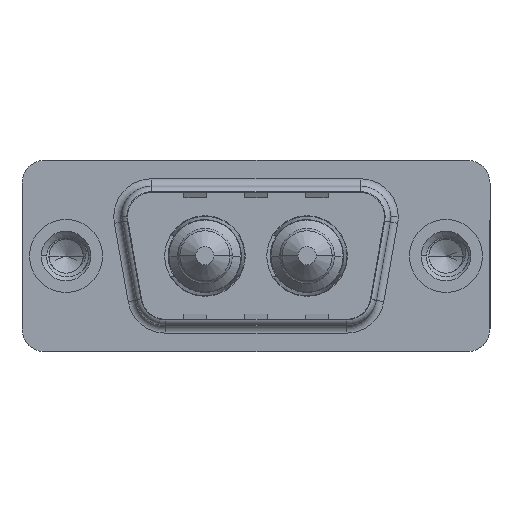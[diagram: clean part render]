
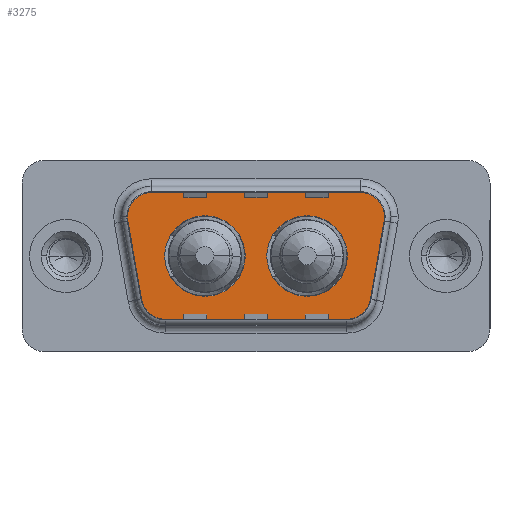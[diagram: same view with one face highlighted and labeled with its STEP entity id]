
A CAD part, top view. The second image highlights one B-rep face of the part: STEP entity #3275.
In plain terms, the highlighted planar face has unit normal (0, 0, 1).
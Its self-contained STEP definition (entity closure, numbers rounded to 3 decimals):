
#17 = EDGE_CURVE ( 'NONE', #4552, #8587, #10843, .T. ) ;
#69 = VECTOR ( 'NONE', #9359, 1000. ) ;
#136 = DIRECTION ( 'NONE',  ( 0., 0., 1. ) ) ;
#342 = CARTESIAN_POINT ( 'NONE',  ( 21.534, 2.553, 0. ) ) ;
#402 = VERTEX_POINT ( 'NONE', #11069 ) ;
#480 = DIRECTION ( 'NONE',  ( -1., 0., 0. ) ) ;
#673 = DIRECTION ( 'NONE',  ( 0.174, -0.985, 0. ) ) ;
#839 = EDGE_CURVE ( 'NONE', #10419, #3076, #1350, .T. ) ;
#845 = ORIENTED_EDGE ( 'NONE', *, *, #6918, .F. ) ;
#943 = CARTESIAN_POINT ( 'NONE',  ( 11.79, 0., 0. ) ) ;
#993 = CARTESIAN_POINT ( 'NONE',  ( 19.564, 2.9, 0. ) ) ;
#1350 = CIRCLE ( 'NONE', #9369, 2. ) ;
#1562 = FACE_BOUND ( 'NONE', #8953, .T. ) ;
#1615 = CARTESIAN_POINT ( 'NONE',  ( 18.541, -4.9, 0. ) ) ;
#1668 = VERTEX_POINT ( 'NONE', #3871 ) ;
#1776 = AXIS2_PLACEMENT_3D ( 'NONE', #9041, #3293, #10035 ) ;
#1849 = CARTESIAN_POINT ( 'NONE',  ( 19.564, 2.9, 0. ) ) ;
#1935 = DIRECTION ( 'NONE',  ( 0., 0., 1. ) ) ;
#1953 = DIRECTION ( 'NONE',  ( 0., 0., 1. ) ) ;
#1958 = DIRECTION ( 'NONE',  ( -1., 0., 0. ) ) ;
#2004 = VECTOR ( 'NONE', #673, 1000. ) ;
#2191 = CARTESIAN_POINT ( 'NONE',  ( 21.564, 2.9, 0. ) ) ;
#2252 = DIRECTION ( 'NONE',  ( 1., 0., 0. ) ) ;
#2276 = LINE ( 'NONE', #2548, #2004 ) ;
#2434 = PLANE ( 'NONE',  #11104 ) ;
#2440 = EDGE_CURVE ( 'NONE', #1668, #12020, #4058, .T. ) ;
#2451 = CARTESIAN_POINT ( 'NONE',  ( 5.436, 2.9, 0. ) ) ;
#2518 = CARTESIAN_POINT ( 'NONE',  ( 13.21, 0., 0. ) ) ;
#2548 = CARTESIAN_POINT ( 'NONE',  ( 3.466, 2.553, 0. ) ) ;
#2599 = EDGE_CURVE ( 'NONE', #3183, #10419, #2601, .T. ) ;
#2601 = LINE ( 'NONE', #342, #69 ) ;
#2719 = EDGE_LOOP ( 'NONE', ( #7186, #10573 ) ) ;
#2853 = EDGE_CURVE ( 'NONE', #3984, #3183, #10420, .T. ) ;
#2894 = VECTOR ( 'NONE', #6659, 1000. ) ;
#3076 = VERTEX_POINT ( 'NONE', #2191 ) ;
#3104 = ORIENTED_EDGE ( 'NONE', *, *, #2440, .T. ) ;
#3174 = LINE ( 'NONE', #8544, #2894 ) ;
#3183 = VERTEX_POINT ( 'NONE', #6648 ) ;
#3245 = DIRECTION ( 'NONE',  ( 0., 0., 1. ) ) ;
#3275 = ADVANCED_FACE ( 'NONE', ( #6599, #1562, #4062 ), #2434, .T. ) ;
#3293 = DIRECTION ( 'NONE',  ( 0., 0., 1. ) ) ;
#3331 = EDGE_LOOP ( 'NONE', ( #6577, #6146, #9523, #11429, #3104, #3980, #6420, #4928, #11741 ) ) ;
#3372 = DIRECTION ( 'NONE',  ( 1., 0., 0. ) ) ;
#3431 = EDGE_CURVE ( 'NONE', #8587, #4552, #5106, .T. ) ;
#3697 = AXIS2_PLACEMENT_3D ( 'NONE', #993, #7604, #1958 ) ;
#3751 = ORIENTED_EDGE ( 'NONE', *, *, #7240, .F. ) ;
#3770 = CARTESIAN_POINT ( 'NONE',  ( 6.49, 0., 0. ) ) ;
#3871 = CARTESIAN_POINT ( 'NONE',  ( 19.564, 4.9, 0. ) ) ;
#3980 = ORIENTED_EDGE ( 'NONE', *, *, #9493, .T. ) ;
#3984 = VERTEX_POINT ( 'NONE', #1615 ) ;
#4058 = LINE ( 'NONE', #11901, #12078 ) ;
#4062 = FACE_OUTER_BOUND ( 'NONE', #3331, .T. ) ;
#4552 = VERTEX_POINT ( 'NONE', #2518 ) ;
#4630 = EDGE_CURVE ( 'NONE', #9684, #402, #2276, .T. ) ;
#4866 = AXIS2_PLACEMENT_3D ( 'NONE', #9092, #9027, #2252 ) ;
#4928 = ORIENTED_EDGE ( 'NONE', *, *, #8724, .T. ) ;
#5028 = AXIS2_PLACEMENT_3D ( 'NONE', #12422, #136, #12000 ) ;
#5081 = DIRECTION ( 'NONE',  ( 0., 0., 1. ) ) ;
#5106 = CIRCLE ( 'NONE', #5028, 2.65 ) ;
#5279 = DIRECTION ( 'NONE',  ( 1., 0., 0. ) ) ;
#5371 = CARTESIAN_POINT ( 'NONE',  ( 5.436, 4.9, 0. ) ) ;
#5622 = VERTEX_POINT ( 'NONE', #7425 ) ;
#5709 = CARTESIAN_POINT ( 'NONE',  ( 18.51, 0., 0. ) ) ;
#6146 = ORIENTED_EDGE ( 'NONE', *, *, #2599, .T. ) ;
#6420 = ORIENTED_EDGE ( 'NONE', *, *, #4630, .T. ) ;
#6577 = ORIENTED_EDGE ( 'NONE', *, *, #2853, .T. ) ;
#6599 = FACE_BOUND ( 'NONE', #2719, .T. ) ;
#6648 = CARTESIAN_POINT ( 'NONE',  ( 20.511, -3.247, 0. ) ) ;
#6659 = DIRECTION ( 'NONE',  ( 1., 0., 0. ) ) ;
#6918 = EDGE_CURVE ( 'NONE', #9177, #9768, #11844, .T. ) ;
#7186 = ORIENTED_EDGE ( 'NONE', *, *, #3431, .F. ) ;
#7240 = EDGE_CURVE ( 'NONE', #9768, #9177, #8775, .T. ) ;
#7425 = CARTESIAN_POINT ( 'NONE',  ( 6.459, -4.9, 0. ) ) ;
#7600 = CARTESIAN_POINT ( 'NONE',  ( 9.14, 0., 0. ) ) ;
#7604 = DIRECTION ( 'NONE',  ( 0., 0., 1. ) ) ;
#7642 = AXIS2_PLACEMENT_3D ( 'NONE', #2451, #9116, #3372 ) ;
#8273 = AXIS2_PLACEMENT_3D ( 'NONE', #7600, #1953, #8588 ) ;
#8376 = CARTESIAN_POINT ( 'NONE',  ( 3.466, 2.553, 0. ) ) ;
#8544 = CARTESIAN_POINT ( 'NONE',  ( 6.459, -4.9, 0. ) ) ;
#8587 = VERTEX_POINT ( 'NONE', #5709 ) ;
#8588 = DIRECTION ( 'NONE',  ( 1., 0., 0. ) ) ;
#8724 = EDGE_CURVE ( 'NONE', #402, #5622, #10914, .T. ) ;
#8775 = CIRCLE ( 'NONE', #8273, 2.65 ) ;
#8953 = EDGE_LOOP ( 'NONE', ( #3751, #845 ) ) ;
#8986 = CARTESIAN_POINT ( 'NONE',  ( 9.14, 0., 0. ) ) ;
#9027 = DIRECTION ( 'NONE',  ( 0., 0., 1. ) ) ;
#9041 = CARTESIAN_POINT ( 'NONE',  ( 6.459, -2.9, 0. ) ) ;
#9092 = CARTESIAN_POINT ( 'NONE',  ( 18.541, -2.9, 0. ) ) ;
#9116 = DIRECTION ( 'NONE',  ( 0., 0., 1. ) ) ;
#9177 = VERTEX_POINT ( 'NONE', #3770 ) ;
#9199 = AXIS2_PLACEMENT_3D ( 'NONE', #11791, #12161, #12397 ) ;
#9349 = CIRCLE ( 'NONE', #7642, 2. ) ;
#9359 = DIRECTION ( 'NONE',  ( 0.174, 0.985, 0. ) ) ;
#9369 = AXIS2_PLACEMENT_3D ( 'NONE', #1849, #1935, #480 ) ;
#9493 = EDGE_CURVE ( 'NONE', #12020, #9684, #9349, .T. ) ;
#9523 = ORIENTED_EDGE ( 'NONE', *, *, #839, .T. ) ;
#9684 = VERTEX_POINT ( 'NONE', #8376 ) ;
#9768 = VERTEX_POINT ( 'NONE', #943 ) ;
#9858 = AXIS2_PLACEMENT_3D ( 'NONE', #8986, #3245, #9994 ) ;
#9994 = DIRECTION ( 'NONE',  ( 1., 0., 0. ) ) ;
#10035 = DIRECTION ( 'NONE',  ( -1., 0., 0. ) ) ;
#10419 = VERTEX_POINT ( 'NONE', #12433 ) ;
#10420 = CIRCLE ( 'NONE', #4866, 2. ) ;
#10573 = ORIENTED_EDGE ( 'NONE', *, *, #17, .F. ) ;
#10583 = CIRCLE ( 'NONE', #3697, 2. ) ;
#10843 = CIRCLE ( 'NONE', #9199, 2.65 ) ;
#10914 = CIRCLE ( 'NONE', #1776, 2. ) ;
#11043 = EDGE_CURVE ( 'NONE', #3076, #1668, #10583, .T. ) ;
#11055 = EDGE_CURVE ( 'NONE', #5622, #3984, #3174, .T. ) ;
#11069 = CARTESIAN_POINT ( 'NONE',  ( 4.489, -3.247, 0. ) ) ;
#11104 = AXIS2_PLACEMENT_3D ( 'NONE', #11717, #5081, #5279 ) ;
#11429 = ORIENTED_EDGE ( 'NONE', *, *, #11043, .T. ) ;
#11658 = DIRECTION ( 'NONE',  ( -1., 0., 0. ) ) ;
#11717 = CARTESIAN_POINT ( 'NONE',  ( 18.541, -2.9, 0. ) ) ;
#11741 = ORIENTED_EDGE ( 'NONE', *, *, #11055, .T. ) ;
#11791 = CARTESIAN_POINT ( 'NONE',  ( 15.86, 0., 0. ) ) ;
#11844 = CIRCLE ( 'NONE', #9858, 2.65 ) ;
#11901 = CARTESIAN_POINT ( 'NONE',  ( 5.436, 4.9, 0. ) ) ;
#12000 = DIRECTION ( 'NONE',  ( 1., 0., 0. ) ) ;
#12020 = VERTEX_POINT ( 'NONE', #5371 ) ;
#12078 = VECTOR ( 'NONE', #11658, 1000. ) ;
#12161 = DIRECTION ( 'NONE',  ( 0., 0., 1. ) ) ;
#12397 = DIRECTION ( 'NONE',  ( 1., 0., 0. ) ) ;
#12422 = CARTESIAN_POINT ( 'NONE',  ( 15.86, 0., 0. ) ) ;
#12433 = CARTESIAN_POINT ( 'NONE',  ( 21.534, 2.553, 0. ) ) ;
